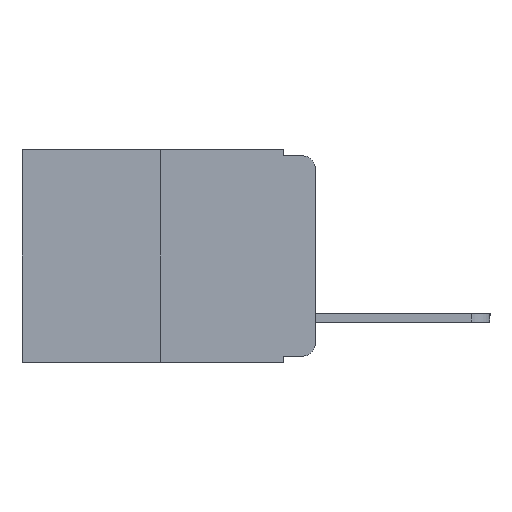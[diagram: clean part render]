
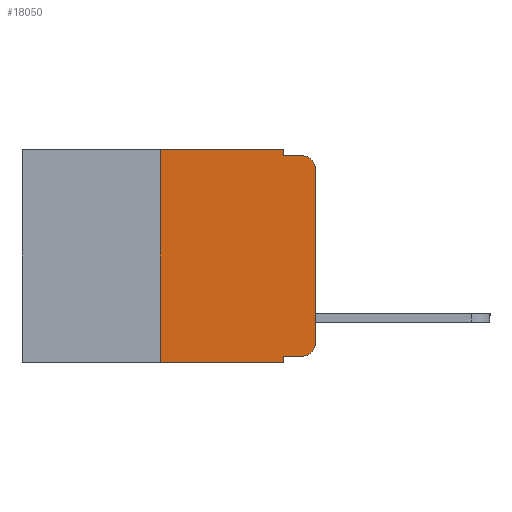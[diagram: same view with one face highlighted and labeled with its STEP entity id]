
A CAD part, left-side view. The second image highlights one B-rep face of the part: STEP entity #18050.
In plain terms, the highlighted planar face has unit normal (-1, 0, 0).
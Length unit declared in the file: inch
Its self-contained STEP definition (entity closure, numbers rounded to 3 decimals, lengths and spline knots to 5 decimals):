
#410 = ORIENTED_EDGE ( 'NONE', *, *, #18353, .T. ) ;
#460 = FACE_OUTER_BOUND ( 'NONE', #2679, .T. ) ;
#693 = EDGE_CURVE ( 'NONE', #5717, #5715, #8880, .T. ) ;
#900 = CARTESIAN_POINT ( 'NONE',  ( 0., 0.051, 0. ) ) ;
#993 = VECTOR ( 'NONE', #15676, 39.37008 ) ;
#1152 = VERTEX_POINT ( 'NONE', #11837 ) ;
#1207 = VERTEX_POINT ( 'NONE', #9541 ) ;
#1739 = EDGE_CURVE ( 'NONE', #5717, #15895, #1911, .T. ) ;
#1885 = DIRECTION ( 'NONE',  ( -1., 0., 0. ) ) ;
#1911 = LINE ( 'NONE', #15523, #5939 ) ;
#2307 = ORIENTED_EDGE ( 'NONE', *, *, #2814, .F. ) ;
#2537 = VECTOR ( 'NONE', #5113, 39.37008 ) ;
#2618 = CARTESIAN_POINT ( 'NONE',  ( 0., 0., 0. ) ) ;
#2679 = EDGE_LOOP ( 'NONE', ( #8012, #18197, #8313, #17794, #16073, #2307, #6710, #5811, #9898, #410 ) ) ;
#2814 = EDGE_CURVE ( 'NONE', #13160, #1207, #13831, .T. ) ;
#2845 = VERTEX_POINT ( 'NONE', #5367 ) ;
#2970 = CARTESIAN_POINT ( 'NONE',  ( 0., 0.473, 0. ) ) ;
#3099 = VECTOR ( 'NONE', #17245, 39.37008 ) ;
#3166 = DIRECTION ( 'NONE',  ( 0., -1., 0. ) ) ;
#3840 = LINE ( 'NONE', #2618, #7202 ) ;
#3890 = EDGE_CURVE ( 'NONE', #12679, #2845, #6983, .T. ) ;
#4500 = AXIS2_PLACEMENT_3D ( 'NONE', #10572, #1885, #12030 ) ;
#4588 = CARTESIAN_POINT ( 'NONE',  ( 0., 0.051, 0. ) ) ;
#4682 = CARTESIAN_POINT ( 'NONE',  ( 0., 0.051, -0.343 ) ) ;
#4870 = EDGE_CURVE ( 'NONE', #2845, #1152, #7854, .T. ) ;
#5113 = DIRECTION ( 'NONE',  ( 0., -1., 0. ) ) ;
#5367 = CARTESIAN_POINT ( 'NONE',  ( 0., 0.051, -0.01 ) ) ;
#5715 = VERTEX_POINT ( 'NONE', #12617 ) ;
#5717 = VERTEX_POINT ( 'NONE', #7005 ) ;
#5811 = ORIENTED_EDGE ( 'NONE', *, *, #1739, .F. ) ;
#5829 = EDGE_CURVE ( 'NONE', #12091, #1152, #10170, .T. ) ;
#5904 = VECTOR ( 'NONE', #3166, 39.37008 ) ;
#5939 = VECTOR ( 'NONE', #9640, 39.37008 ) ;
#6397 = AXIS2_PLACEMENT_3D ( 'NONE', #16781, #8429, #18170 ) ;
#6433 = DIRECTION ( 'NONE',  ( 0., 0., -1. ) ) ;
#6710 = ORIENTED_EDGE ( 'NONE', *, *, #11113, .T. ) ;
#6768 = EDGE_CURVE ( 'NONE', #17242, #12091, #3840, .T. ) ;
#6772 = CARTESIAN_POINT ( 'NONE',  ( 0., 0.25, 0. ) ) ;
#6867 = CARTESIAN_POINT ( 'NONE',  ( 0., 0.051, -0.333 ) ) ;
#6983 = LINE ( 'NONE', #4588, #3099 ) ;
#7005 = CARTESIAN_POINT ( 'NONE',  ( 0., 0.051, -0.333 ) ) ;
#7202 = VECTOR ( 'NONE', #18185, 39.37008 ) ;
#7341 = LINE ( 'NONE', #2970, #10166 ) ;
#7854 = LINE ( 'NONE', #7912, #2537 ) ;
#7912 = CARTESIAN_POINT ( 'NONE',  ( 0., 0.051, -0.01 ) ) ;
#8012 = ORIENTED_EDGE ( 'NONE', *, *, #6768, .T. ) ;
#8099 = CARTESIAN_POINT ( 'NONE',  ( 0., 0., -0.03 ) ) ;
#8209 = CIRCLE ( 'NONE', #6397, 0.02 ) ;
#8313 = ORIENTED_EDGE ( 'NONE', *, *, #4870, .F. ) ;
#8429 = DIRECTION ( 'NONE',  ( -1., 0., 0. ) ) ;
#8581 = EDGE_CURVE ( 'NONE', #1207, #12679, #7341, .T. ) ;
#8880 = LINE ( 'NONE', #6867, #993 ) ;
#9228 = PLANE ( 'NONE',  #12444 ) ;
#9541 = CARTESIAN_POINT ( 'NONE',  ( 0., 0.25, 0. ) ) ;
#9640 = DIRECTION ( 'NONE',  ( 0., 0., -1. ) ) ;
#9898 = ORIENTED_EDGE ( 'NONE', *, *, #693, .T. ) ;
#10051 = VECTOR ( 'NONE', #12457, 39.37008 ) ;
#10166 = VECTOR ( 'NONE', #14323, 39.37008 ) ;
#10170 = CIRCLE ( 'NONE', #4500, 0.02 ) ;
#10572 = CARTESIAN_POINT ( 'NONE',  ( 0., 0.02, -0.03 ) ) ;
#11113 = EDGE_CURVE ( 'NONE', #13160, #15895, #17085, .T. ) ;
#11837 = CARTESIAN_POINT ( 'NONE',  ( 0., 0.02, -0.01 ) ) ;
#12030 = DIRECTION ( 'NONE',  ( 0., 0., -1. ) ) ;
#12056 = CARTESIAN_POINT ( 'NONE',  ( 0., 0.473, 0. ) ) ;
#12091 = VERTEX_POINT ( 'NONE', #8099 ) ;
#12444 = AXIS2_PLACEMENT_3D ( 'NONE', #12056, #14852, #6433 ) ;
#12457 = DIRECTION ( 'NONE',  ( 0., 0., 1. ) ) ;
#12617 = CARTESIAN_POINT ( 'NONE',  ( 0., 0.02, -0.333 ) ) ;
#12679 = VERTEX_POINT ( 'NONE', #900 ) ;
#13160 = VERTEX_POINT ( 'NONE', #17298 ) ;
#13200 = CARTESIAN_POINT ( 'NONE',  ( 0., 0., -0.313 ) ) ;
#13831 = LINE ( 'NONE', #6772, #10051 ) ;
#14323 = DIRECTION ( 'NONE',  ( 0., -1., 0. ) ) ;
#14852 = DIRECTION ( 'NONE',  ( 1., 0., 0. ) ) ;
#15523 = CARTESIAN_POINT ( 'NONE',  ( 0., 0.051, 0. ) ) ;
#15676 = DIRECTION ( 'NONE',  ( 0., -1., 0. ) ) ;
#15895 = VERTEX_POINT ( 'NONE', #4682 ) ;
#16073 = ORIENTED_EDGE ( 'NONE', *, *, #8581, .F. ) ;
#16781 = CARTESIAN_POINT ( 'NONE',  ( 0., 0.02, -0.313 ) ) ;
#17085 = LINE ( 'NONE', #17330, #5904 ) ;
#17242 = VERTEX_POINT ( 'NONE', #13200 ) ;
#17245 = DIRECTION ( 'NONE',  ( 0., 0., -1. ) ) ;
#17298 = CARTESIAN_POINT ( 'NONE',  ( 0., 0.25, -0.343 ) ) ;
#17330 = CARTESIAN_POINT ( 'NONE',  ( 0., 0.473, -0.343 ) ) ;
#17794 = ORIENTED_EDGE ( 'NONE', *, *, #3890, .F. ) ;
#18050 = ADVANCED_FACE ( 'NONE', ( #460 ), #9228, .F. ) ;
#18170 = DIRECTION ( 'NONE',  ( 0., 0., -1. ) ) ;
#18185 = DIRECTION ( 'NONE',  ( 0., 0., 1. ) ) ;
#18197 = ORIENTED_EDGE ( 'NONE', *, *, #5829, .T. ) ;
#18353 = EDGE_CURVE ( 'NONE', #5715, #17242, #8209, .T. ) ;
